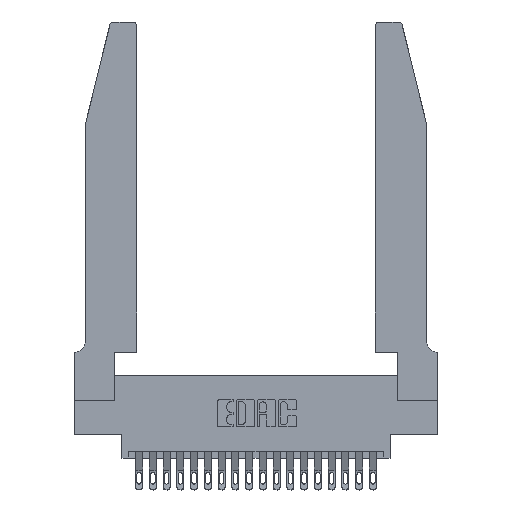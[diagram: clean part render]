
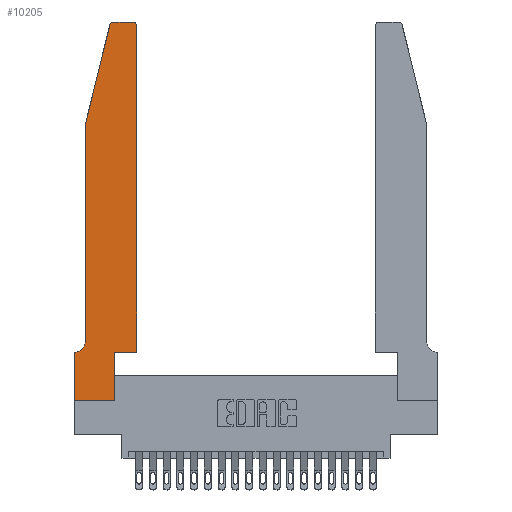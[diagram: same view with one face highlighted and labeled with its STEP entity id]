
A CAD part, top view. The second image highlights one B-rep face of the part: STEP entity #10205.
In plain terms, the highlighted planar face has unit normal (0, 0, 1).
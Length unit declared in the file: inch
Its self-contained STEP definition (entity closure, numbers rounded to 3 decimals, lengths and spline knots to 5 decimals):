
#46 = VECTOR ( 'NONE', #2156, 39.37008 ) ;
#168 = CARTESIAN_POINT ( 'NONE',  ( 0.4505, 0.35, 0.37 ) ) ;
#209 = FACE_OUTER_BOUND ( 'NONE', #19329, .T. ) ;
#1416 = AXIS2_PLACEMENT_3D ( 'NONE', #5628, #3856, #17858 ) ;
#1927 = CARTESIAN_POINT ( 'NONE',  ( 0., 0., 0.37 ) ) ;
#2047 = AXIS2_PLACEMENT_3D ( 'NONE', #6514, #18570, #8255 ) ;
#2156 = DIRECTION ( 'NONE',  ( 0., -1., 0. ) ) ;
#2311 = LINE ( 'NONE', #168, #14155 ) ;
#2464 = DIRECTION ( 'NONE',  ( -1., 0., 0. ) ) ;
#2505 = VERTEX_POINT ( 'NONE', #19284 ) ;
#2889 = EDGE_CURVE ( 'NONE', #3067, #11324, #14284, .T. ) ;
#3067 = VERTEX_POINT ( 'NONE', #5391 ) ;
#3210 = VECTOR ( 'NONE', #4670, 39.37008 ) ;
#3218 = VECTOR ( 'NONE', #20628, 39.37008 ) ;
#3702 = VECTOR ( 'NONE', #19810, 39.37008 ) ;
#3856 = DIRECTION ( 'NONE',  ( 0., 0., 1. ) ) ;
#4265 = LINE ( 'NONE', #18063, #3702 ) ;
#4437 = EDGE_CURVE ( 'NONE', #16254, #11331, #13113, .T. ) ;
#4670 = DIRECTION ( 'NONE',  ( 0., -1., 0. ) ) ;
#4783 = AXIS2_PLACEMENT_3D ( 'NONE', #18927, #8608, #20651 ) ;
#5074 = VERTEX_POINT ( 'NONE', #21870 ) ;
#5376 = VERTEX_POINT ( 'NONE', #5746 ) ;
#5391 = CARTESIAN_POINT ( 'NONE',  ( 0.4205, 2.75, 0.37 ) ) ;
#5628 = CARTESIAN_POINT ( 'NONE',  ( 0.284, 2.72, 0.37 ) ) ;
#5746 = CARTESIAN_POINT ( 'NONE',  ( 0.0055, 0.35, 0.37 ) ) ;
#5869 = VECTOR ( 'NONE', #2464, 39.37008 ) ;
#6272 = CARTESIAN_POINT ( 'NONE',  ( 0., 0., 0.37 ) ) ;
#6514 = CARTESIAN_POINT ( 'NONE',  ( 0.4205, 2.72, 0.37 ) ) ;
#6555 = EDGE_CURVE ( 'NONE', #2505, #16159, #2311, .T. ) ;
#6562 = CIRCLE ( 'NONE', #2047, 0.03 ) ;
#7024 = LINE ( 'NONE', #6272, #15698 ) ;
#7097 = EDGE_CURVE ( 'NONE', #7299, #12613, #15197, .T. ) ;
#7299 = VERTEX_POINT ( 'NONE', #11947 ) ;
#7872 = DIRECTION ( 'NONE',  ( 1., 0., 0. ) ) ;
#7911 = ORIENTED_EDGE ( 'NONE', *, *, #21599, .T. ) ;
#8116 = CARTESIAN_POINT ( 'NONE',  ( 0., 0., 0.37 ) ) ;
#8255 = DIRECTION ( 'NONE',  ( 1., 0., 0. ) ) ;
#8289 = DIRECTION ( 'NONE',  ( 0., 1., 0. ) ) ;
#8443 = ORIENTED_EDGE ( 'NONE', *, *, #11631, .T. ) ;
#8608 = DIRECTION ( 'NONE',  ( 0., 0., -1. ) ) ;
#9358 = EDGE_CURVE ( 'NONE', #11324, #15393, #13208, .T. ) ;
#9489 = EDGE_CURVE ( 'NONE', #5376, #16254, #16160, .T. ) ;
#9499 = CARTESIAN_POINT ( 'NONE',  ( 0.4505, 0.35, 0.37 ) ) ;
#9939 = CARTESIAN_POINT ( 'NONE',  ( 0.4505, 2.72, 0.37 ) ) ;
#10205 = ADVANCED_FACE ( 'NONE', ( #209 ), #14790, .T. ) ;
#10423 = ORIENTED_EDGE ( 'NONE', *, *, #6555, .T. ) ;
#10767 = ORIENTED_EDGE ( 'NONE', *, *, #2889, .T. ) ;
#10791 = DIRECTION ( 'NONE',  ( 1., 0., 0. ) ) ;
#10970 = ORIENTED_EDGE ( 'NONE', *, *, #16149, .T. ) ;
#10976 = CARTESIAN_POINT ( 'NONE',  ( 0.0755, 2., 0.37 ) ) ;
#11302 = ORIENTED_EDGE ( 'NONE', *, *, #20883, .T. ) ;
#11324 = VERTEX_POINT ( 'NONE', #17572 ) ;
#11331 = VERTEX_POINT ( 'NONE', #1927 ) ;
#11631 = EDGE_CURVE ( 'NONE', #15393, #7299, #12578, .T. ) ;
#11947 = CARTESIAN_POINT ( 'NONE',  ( 0.0755, 2., 0.37 ) ) ;
#11998 = VERTEX_POINT ( 'NONE', #9939 ) ;
#12291 = CIRCLE ( 'NONE', #4783, 0.07 ) ;
#12578 = LINE ( 'NONE', #18830, #3218 ) ;
#12613 = VERTEX_POINT ( 'NONE', #22431 ) ;
#13113 = LINE ( 'NONE', #8116, #3210 ) ;
#13208 = CIRCLE ( 'NONE', #1416, 0.03 ) ;
#13219 = CARTESIAN_POINT ( 'NONE',  ( 0., 0.35, 0.37 ) ) ;
#13456 = ORIENTED_EDGE ( 'NONE', *, *, #4437, .T. ) ;
#13509 = DIRECTION ( 'NONE',  ( -1., 0., 0. ) ) ;
#13848 = AXIS2_PLACEMENT_3D ( 'NONE', #16500, #18197, #7872 ) ;
#13853 = LINE ( 'NONE', #16907, #22394 ) ;
#13887 = CARTESIAN_POINT ( 'NONE',  ( 0.2605, 2.75, 0.37 ) ) ;
#14155 = VECTOR ( 'NONE', #10791, 39.37008 ) ;
#14284 = LINE ( 'NONE', #13887, #15345 ) ;
#14335 = CARTESIAN_POINT ( 'NONE',  ( 0.25487, 2.72718, 0.37 ) ) ;
#14396 = EDGE_CURVE ( 'NONE', #5074, #2505, #13853, .T. ) ;
#14606 = ORIENTED_EDGE ( 'NONE', *, *, #9358, .T. ) ;
#14790 = PLANE ( 'NONE',  #13848 ) ;
#15004 = DIRECTION ( 'NONE',  ( 1., 0., 0. ) ) ;
#15197 = LINE ( 'NONE', #10976, #46 ) ;
#15345 = VECTOR ( 'NONE', #13509, 39.37008 ) ;
#15393 = VERTEX_POINT ( 'NONE', #14335 ) ;
#15698 = VECTOR ( 'NONE', #15004, 39.37008 ) ;
#16149 = EDGE_CURVE ( 'NONE', #16159, #11998, #4265, .T. ) ;
#16159 = VERTEX_POINT ( 'NONE', #9499 ) ;
#16160 = LINE ( 'NONE', #21531, #5869 ) ;
#16254 = VERTEX_POINT ( 'NONE', #13219 ) ;
#16500 = CARTESIAN_POINT ( 'NONE',  ( 0., 0.35, 0.37 ) ) ;
#16826 = EDGE_CURVE ( 'NONE', #11331, #5074, #7024, .T. ) ;
#16907 = CARTESIAN_POINT ( 'NONE',  ( 0.2865, 0.35, 0.37 ) ) ;
#17572 = CARTESIAN_POINT ( 'NONE',  ( 0.284, 2.75, 0.37 ) ) ;
#17858 = DIRECTION ( 'NONE',  ( 1., 0., 0. ) ) ;
#18063 = CARTESIAN_POINT ( 'NONE',  ( 0.4505, 0.35, 0.37 ) ) ;
#18197 = DIRECTION ( 'NONE',  ( 0., 0., 1. ) ) ;
#18570 = DIRECTION ( 'NONE',  ( 0., 0., 1. ) ) ;
#18742 = ORIENTED_EDGE ( 'NONE', *, *, #14396, .T. ) ;
#18830 = CARTESIAN_POINT ( 'NONE',  ( 0.0755, 2., 0.37 ) ) ;
#18927 = CARTESIAN_POINT ( 'NONE',  ( 0.0055, 0.42, 0.37 ) ) ;
#19284 = CARTESIAN_POINT ( 'NONE',  ( 0.2865, 0.35, 0.37 ) ) ;
#19329 = EDGE_LOOP ( 'NONE', ( #10767, #14606, #8443, #20258, #7911, #21588, #13456, #19615, #18742, #10423, #10970, #11302 ) ) ;
#19615 = ORIENTED_EDGE ( 'NONE', *, *, #16826, .T. ) ;
#19810 = DIRECTION ( 'NONE',  ( 0., 1., 0. ) ) ;
#20258 = ORIENTED_EDGE ( 'NONE', *, *, #7097, .T. ) ;
#20628 = DIRECTION ( 'NONE',  ( -0.239, -0.971, 0. ) ) ;
#20651 = DIRECTION ( 'NONE',  ( -1., 0., 0. ) ) ;
#20883 = EDGE_CURVE ( 'NONE', #11998, #3067, #6562, .T. ) ;
#21531 = CARTESIAN_POINT ( 'NONE',  ( 0.0755, 0.35, 0.37 ) ) ;
#21588 = ORIENTED_EDGE ( 'NONE', *, *, #9489, .T. ) ;
#21599 = EDGE_CURVE ( 'NONE', #12613, #5376, #12291, .T. ) ;
#21870 = CARTESIAN_POINT ( 'NONE',  ( 0.2865, 0., 0.37 ) ) ;
#22394 = VECTOR ( 'NONE', #8289, 39.37008 ) ;
#22431 = CARTESIAN_POINT ( 'NONE',  ( 0.0755, 0.42, 0.37 ) ) ;
